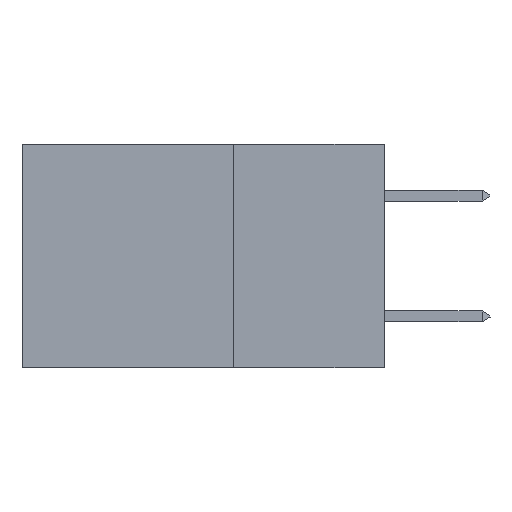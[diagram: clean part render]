
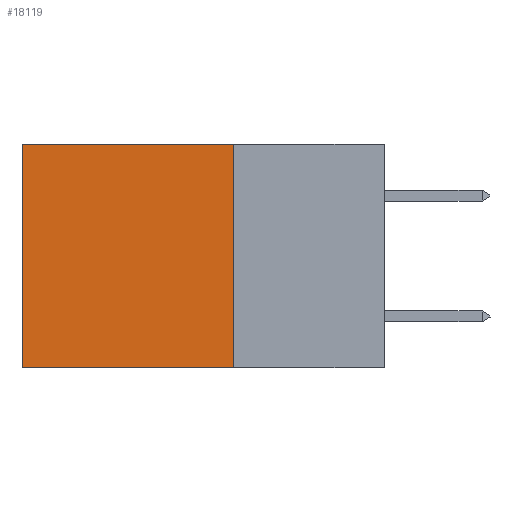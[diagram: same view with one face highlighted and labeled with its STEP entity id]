
A CAD part, left-side view. The second image highlights one B-rep face of the part: STEP entity #18119.
In plain terms, the highlighted planar face has unit normal (-1, 0, 0).
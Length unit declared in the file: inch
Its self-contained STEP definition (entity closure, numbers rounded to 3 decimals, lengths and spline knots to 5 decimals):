
#486 = LINE ( 'NONE', #20114, #12920 ) ;
#784 = ORIENTED_EDGE ( 'NONE', *, *, #15807, .T. ) ;
#1028 = VERTEX_POINT ( 'NONE', #1683 ) ;
#1447 = ORIENTED_EDGE ( 'NONE', *, *, #6549, .F. ) ;
#1683 = CARTESIAN_POINT ( 'NONE',  ( 0.2875, 0.25, -0.37 ) ) ;
#3559 = LINE ( 'NONE', #34485, #36724 ) ;
#3735 = CARTESIAN_POINT ( 'NONE',  ( 0.2875, 0.25, -0.37 ) ) ;
#3959 = CARTESIAN_POINT ( 'NONE',  ( 0.2875, 0.6, 0. ) ) ;
#4868 = DIRECTION ( 'NONE',  ( 0., 0., -1. ) ) ;
#5430 = ORIENTED_EDGE ( 'NONE', *, *, #10263, .T. ) ;
#6182 = LINE ( 'NONE', #37532, #31563 ) ;
#6549 = EDGE_CURVE ( 'NONE', #1028, #34487, #13942, .T. ) ;
#7368 = EDGE_LOOP ( 'NONE', ( #5430, #1447, #41246, #784 ) ) ;
#8165 = FACE_OUTER_BOUND ( 'NONE', #7368, .T. ) ;
#10263 = EDGE_CURVE ( 'NONE', #28867, #34487, #486, .T. ) ;
#10713 = DIRECTION ( 'NONE',  ( 0., 1., 0. ) ) ;
#12920 = VECTOR ( 'NONE', #13517, 39.37008 ) ;
#13517 = DIRECTION ( 'NONE',  ( 0., 0., -1. ) ) ;
#13942 = LINE ( 'NONE', #3735, #16499 ) ;
#15807 = EDGE_CURVE ( 'NONE', #32892, #28867, #6182, .T. ) ;
#16134 = AXIS2_PLACEMENT_3D ( 'NONE', #41577, #34821, #4868 ) ;
#16499 = VECTOR ( 'NONE', #10713, 39.37008 ) ;
#18119 = ADVANCED_FACE ( 'NONE', ( #8165 ), #31335, .F. ) ;
#20114 = CARTESIAN_POINT ( 'NONE',  ( 0.2875, 0.6, 0. ) ) ;
#21907 = CARTESIAN_POINT ( 'NONE',  ( 0.2875, 0.6, -0.37 ) ) ;
#28867 = VERTEX_POINT ( 'NONE', #3959 ) ;
#31335 = PLANE ( 'NONE',  #16134 ) ;
#31563 = VECTOR ( 'NONE', #34319, 39.37008 ) ;
#32248 = EDGE_CURVE ( 'NONE', #32892, #1028, #3559, .T. ) ;
#32892 = VERTEX_POINT ( 'NONE', #37833 ) ;
#34319 = DIRECTION ( 'NONE',  ( 0., 1., 0. ) ) ;
#34485 = CARTESIAN_POINT ( 'NONE',  ( 0.2875, 0.25, 0. ) ) ;
#34487 = VERTEX_POINT ( 'NONE', #21907 ) ;
#34821 = DIRECTION ( 'NONE',  ( 1., 0., 0. ) ) ;
#36724 = VECTOR ( 'NONE', #41263, 39.37008 ) ;
#37532 = CARTESIAN_POINT ( 'NONE',  ( 0.2875, 0.25, 0. ) ) ;
#37833 = CARTESIAN_POINT ( 'NONE',  ( 0.2875, 0.25, 0. ) ) ;
#41246 = ORIENTED_EDGE ( 'NONE', *, *, #32248, .F. ) ;
#41263 = DIRECTION ( 'NONE',  ( 0., 0., -1. ) ) ;
#41577 = CARTESIAN_POINT ( 'NONE',  ( 0.2875, 0.25, 0. ) ) ;
